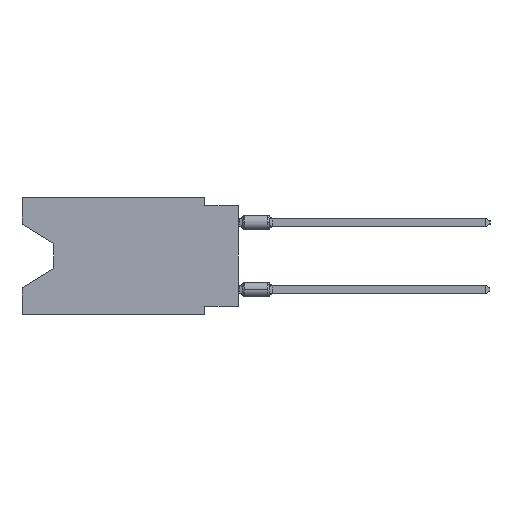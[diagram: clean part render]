
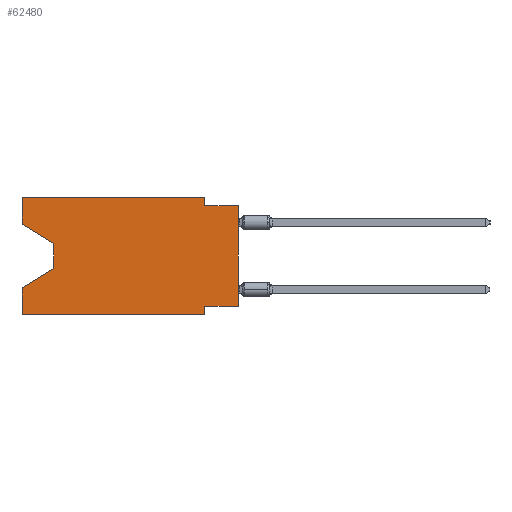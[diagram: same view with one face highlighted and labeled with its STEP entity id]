
A CAD part, left-side view. The second image highlights one B-rep face of the part: STEP entity #62480.
In plain terms, the highlighted planar face has unit normal (-1, 0, 0).
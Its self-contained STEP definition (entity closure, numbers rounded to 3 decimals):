
#719 = VECTOR ( 'NONE', #18138, 1000. ) ;
#862 = CARTESIAN_POINT ( 'NONE',  ( 0., 0., -8.255 ) ) ;
#946 = VERTEX_POINT ( 'NONE', #36964 ) ;
#1460 = CARTESIAN_POINT ( 'NONE',  ( 0., 16.383, -8.89 ) ) ;
#2422 = CARTESIAN_POINT ( 'NONE',  ( 0., 16.383, 0. ) ) ;
#2427 = LINE ( 'NONE', #31409, #43908 ) ;
#3017 = CARTESIAN_POINT ( 'NONE',  ( 0., 16.383, 0. ) ) ;
#5208 = VECTOR ( 'NONE', #28338, 1000. ) ;
#5330 = LINE ( 'NONE', #862, #62084 ) ;
#5463 = DIRECTION ( 'NONE',  ( 0., -0.855, -0.519 ) ) ;
#5534 = DIRECTION ( 'NONE',  ( 0., -1., 0. ) ) ;
#7514 = DIRECTION ( 'NONE',  ( 0., -1., 0. ) ) ;
#7606 = EDGE_CURVE ( 'NONE', #946, #62271, #50687, .T. ) ;
#7786 = DIRECTION ( 'NONE',  ( 1., 0., 0. ) ) ;
#8688 = EDGE_CURVE ( 'NONE', #19505, #22289, #29278, .T. ) ;
#8950 = VERTEX_POINT ( 'NONE', #41959 ) ;
#9189 = DIRECTION ( 'NONE',  ( 0., 0., 1. ) ) ;
#9218 = CARTESIAN_POINT ( 'NONE',  ( 0., 2.54, -8.89 ) ) ;
#9755 = ORIENTED_EDGE ( 'NONE', *, *, #36806, .F. ) ;
#10474 = EDGE_CURVE ( 'NONE', #55806, #41981, #31714, .T. ) ;
#11812 = CARTESIAN_POINT ( 'NONE',  ( 0., 0., -0.635 ) ) ;
#13724 = ORIENTED_EDGE ( 'NONE', *, *, #56443, .T. ) ;
#14289 = LINE ( 'NONE', #53768, #37567 ) ;
#14950 = DIRECTION ( 'NONE',  ( 0., 0., -1. ) ) ;
#15036 = EDGE_CURVE ( 'NONE', #21650, #59622, #39163, .T. ) ;
#16094 = ORIENTED_EDGE ( 'NONE', *, *, #15036, .F. ) ;
#16273 = VECTOR ( 'NONE', #14950, 1000. ) ;
#17252 = ORIENTED_EDGE ( 'NONE', *, *, #10474, .F. ) ;
#18138 = DIRECTION ( 'NONE',  ( 0., -1., 0. ) ) ;
#18225 = LINE ( 'NONE', #32249, #59447 ) ;
#18305 = EDGE_CURVE ( 'NONE', #62271, #41981, #18225, .T. ) ;
#18319 = DIRECTION ( 'NONE',  ( 0., 0., 1. ) ) ;
#19505 = VERTEX_POINT ( 'NONE', #28108 ) ;
#20133 = LINE ( 'NONE', #58028, #55649 ) ;
#21389 = DIRECTION ( 'NONE',  ( 0., 0., -1. ) ) ;
#21650 = VERTEX_POINT ( 'NONE', #25322 ) ;
#21685 = VECTOR ( 'NONE', #5534, 1000. ) ;
#22289 = VERTEX_POINT ( 'NONE', #56744 ) ;
#22569 = ORIENTED_EDGE ( 'NONE', *, *, #55478, .F. ) ;
#22918 = LINE ( 'NONE', #42352, #719 ) ;
#25322 = CARTESIAN_POINT ( 'NONE',  ( 0., 2.54, -8.255 ) ) ;
#25542 = CARTESIAN_POINT ( 'NONE',  ( 0., 13.97, -3.505 ) ) ;
#25939 = ORIENTED_EDGE ( 'NONE', *, *, #26774, .F. ) ;
#26774 = EDGE_CURVE ( 'NONE', #22289, #30590, #22918, .T. ) ;
#27221 = DIRECTION ( 'NONE',  ( 0., 0., -1. ) ) ;
#28108 = CARTESIAN_POINT ( 'NONE',  ( 0., 2.54, 0. ) ) ;
#28338 = DIRECTION ( 'NONE',  ( 0., 0., -1. ) ) ;
#29278 = LINE ( 'NONE', #39474, #16273 ) ;
#29541 = ORIENTED_EDGE ( 'NONE', *, *, #7606, .T. ) ;
#30283 = VECTOR ( 'NONE', #18319, 1000. ) ;
#30370 = CARTESIAN_POINT ( 'NONE',  ( 0., 16.383, 0. ) ) ;
#30590 = VERTEX_POINT ( 'NONE', #11812 ) ;
#31409 = CARTESIAN_POINT ( 'NONE',  ( 0., 16.383, -8.89 ) ) ;
#31714 = LINE ( 'NONE', #2422, #30283 ) ;
#31979 = FACE_OUTER_BOUND ( 'NONE', #32075, .T. ) ;
#32075 = EDGE_LOOP ( 'NONE', ( #13724, #29541, #44359, #17252, #50953, #16094, #22569, #60537, #25939, #36763, #49268, #9755 ) ) ;
#32249 = CARTESIAN_POINT ( 'NONE',  ( 0., 13.97, -5.385 ) ) ;
#32302 = PLANE ( 'NONE',  #36728 ) ;
#32867 = CARTESIAN_POINT ( 'NONE',  ( 0., 0., -8.255 ) ) ;
#36728 = AXIS2_PLACEMENT_3D ( 'NONE', #51414, #7786, #27221 ) ;
#36763 = ORIENTED_EDGE ( 'NONE', *, *, #8688, .F. ) ;
#36806 = EDGE_CURVE ( 'NONE', #8950, #45503, #41280, .T. ) ;
#36964 = CARTESIAN_POINT ( 'NONE',  ( 0., 13.97, -3.505 ) ) ;
#37567 = VECTOR ( 'NONE', #9189, 1000. ) ;
#38637 = EDGE_CURVE ( 'NONE', #45503, #19505, #48851, .T. ) ;
#38959 = VERTEX_POINT ( 'NONE', #32867 ) ;
#39163 = LINE ( 'NONE', #9218, #5208 ) ;
#39474 = CARTESIAN_POINT ( 'NONE',  ( 0., 2.54, 0. ) ) ;
#41280 = LINE ( 'NONE', #3017, #49092 ) ;
#41378 = CARTESIAN_POINT ( 'NONE',  ( 0., 16.383, 0. ) ) ;
#41959 = CARTESIAN_POINT ( 'NONE',  ( 0., 16.383, -2.038 ) ) ;
#41981 = VERTEX_POINT ( 'NONE', #55002 ) ;
#42070 = EDGE_CURVE ( 'NONE', #55806, #59622, #2427, .T. ) ;
#42352 = CARTESIAN_POINT ( 'NONE',  ( 0., 0., -0.635 ) ) ;
#43908 = VECTOR ( 'NONE', #7514, 1000. ) ;
#44359 = ORIENTED_EDGE ( 'NONE', *, *, #18305, .T. ) ;
#45503 = VERTEX_POINT ( 'NONE', #41378 ) ;
#47789 = DIRECTION ( 'NONE',  ( 0., 1., 0. ) ) ;
#47864 = CARTESIAN_POINT ( 'NONE',  ( 0., 2.54, -8.89 ) ) ;
#48851 = LINE ( 'NONE', #30370, #21685 ) ;
#49092 = VECTOR ( 'NONE', #60713, 1000. ) ;
#49268 = ORIENTED_EDGE ( 'NONE', *, *, #38637, .F. ) ;
#50612 = VECTOR ( 'NONE', #21389, 1000. ) ;
#50687 = LINE ( 'NONE', #25542, #50612 ) ;
#50953 = ORIENTED_EDGE ( 'NONE', *, *, #42070, .T. ) ;
#51414 = CARTESIAN_POINT ( 'NONE',  ( 0., 16.383, 0. ) ) ;
#53768 = CARTESIAN_POINT ( 'NONE',  ( 0., 0., 0. ) ) ;
#54355 = EDGE_CURVE ( 'NONE', #38959, #30590, #14289, .T. ) ;
#55002 = CARTESIAN_POINT ( 'NONE',  ( 0., 16.383, -6.852 ) ) ;
#55478 = EDGE_CURVE ( 'NONE', #38959, #21650, #5330, .T. ) ;
#55649 = VECTOR ( 'NONE', #5463, 1000. ) ;
#55806 = VERTEX_POINT ( 'NONE', #1460 ) ;
#56191 = CARTESIAN_POINT ( 'NONE',  ( 0., 13.97, -5.385 ) ) ;
#56443 = EDGE_CURVE ( 'NONE', #8950, #946, #20133, .T. ) ;
#56744 = CARTESIAN_POINT ( 'NONE',  ( 0., 2.54, -0.635 ) ) ;
#58028 = CARTESIAN_POINT ( 'NONE',  ( 0., 16.383, -2.038 ) ) ;
#59447 = VECTOR ( 'NONE', #60939, 1000. ) ;
#59622 = VERTEX_POINT ( 'NONE', #47864 ) ;
#60537 = ORIENTED_EDGE ( 'NONE', *, *, #54355, .T. ) ;
#60713 = DIRECTION ( 'NONE',  ( 0., 0., 1. ) ) ;
#60939 = DIRECTION ( 'NONE',  ( 0., 0.855, -0.519 ) ) ;
#62084 = VECTOR ( 'NONE', #47789, 1000. ) ;
#62271 = VERTEX_POINT ( 'NONE', #56191 ) ;
#62480 = ADVANCED_FACE ( 'NONE', ( #31979 ), #32302, .F. ) ;
